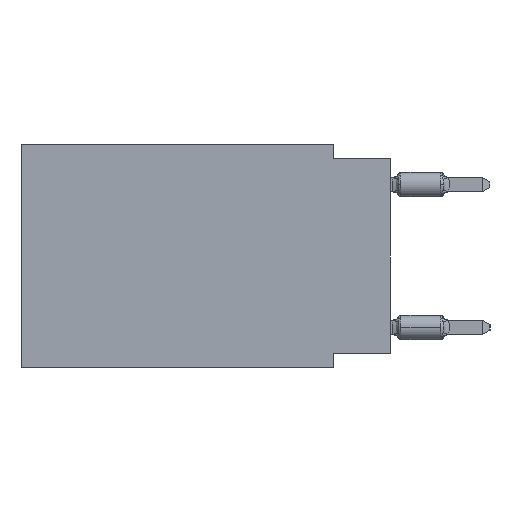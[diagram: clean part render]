
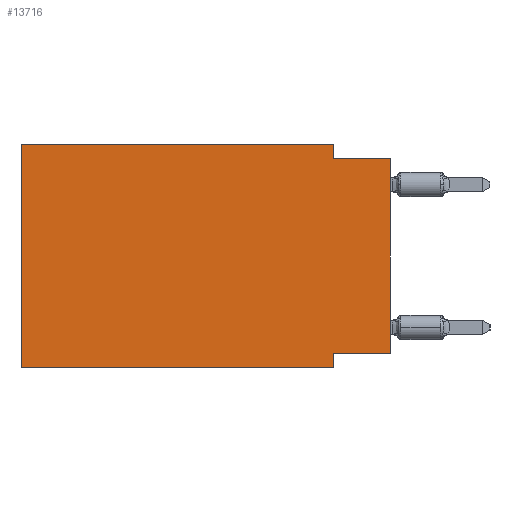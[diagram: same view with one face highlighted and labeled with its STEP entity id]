
A CAD part, left-side view. The second image highlights one B-rep face of the part: STEP entity #13716.
In plain terms, the highlighted planar face has unit normal (-1, 0, 0).
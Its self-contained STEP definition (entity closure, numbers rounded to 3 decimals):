
#2653 = VECTOR ( 'NONE', #44241, 1000. ) ;
#2977 = VECTOR ( 'NONE', #38509, 1000. ) ;
#3052 = VERTEX_POINT ( 'NONE', #7721 ) ;
#3448 = LINE ( 'NONE', #23292, #17995 ) ;
#3545 = ORIENTED_EDGE ( 'NONE', *, *, #43827, .F. ) ;
#4111 = AXIS2_PLACEMENT_3D ( 'NONE', #21947, #48461, #5827 ) ;
#4269 = VERTEX_POINT ( 'NONE', #36253 ) ;
#5827 = DIRECTION ( 'NONE',  ( 0., 0., -1. ) ) ;
#6139 = LINE ( 'NONE', #10091, #47481 ) ;
#7126 = DIRECTION ( 'NONE',  ( 0., -1., 0. ) ) ;
#7233 = VERTEX_POINT ( 'NONE', #31662 ) ;
#7721 = CARTESIAN_POINT ( 'NONE',  ( 0., 0., -9.271 ) ) ;
#7916 = CARTESIAN_POINT ( 'NONE',  ( 0., 0., 0. ) ) ;
#8437 = LINE ( 'NONE', #7916, #37009 ) ;
#9662 = DIRECTION ( 'NONE',  ( 0., -1., 0. ) ) ;
#9807 = FACE_OUTER_BOUND ( 'NONE', #15018, .T. ) ;
#10091 = CARTESIAN_POINT ( 'NONE',  ( 0., 0., -0.635 ) ) ;
#10101 = ORIENTED_EDGE ( 'NONE', *, *, #42262, .T. ) ;
#10187 = VECTOR ( 'NONE', #20282, 1000. ) ;
#10326 = CARTESIAN_POINT ( 'NONE',  ( 0., 16.383, -9.906 ) ) ;
#10565 = VERTEX_POINT ( 'NONE', #40290 ) ;
#13209 = ORIENTED_EDGE ( 'NONE', *, *, #31185, .F. ) ;
#13498 = EDGE_CURVE ( 'NONE', #15154, #10565, #43044, .T. ) ;
#13716 = ADVANCED_FACE ( 'NONE', ( #9807 ), #42030, .F. ) ;
#13750 = ORIENTED_EDGE ( 'NONE', *, *, #44589, .T. ) ;
#13898 = ORIENTED_EDGE ( 'NONE', *, *, #13498, .F. ) ;
#15018 = EDGE_LOOP ( 'NONE', ( #13750, #30929, #37680, #13898, #39206, #10101, #13209, #3545 ) ) ;
#15154 = VERTEX_POINT ( 'NONE', #19608 ) ;
#17995 = VECTOR ( 'NONE', #43879, 1000. ) ;
#18078 = VECTOR ( 'NONE', #9662, 1000. ) ;
#19608 = CARTESIAN_POINT ( 'NONE',  ( 0., 16.383, 0. ) ) ;
#20282 = DIRECTION ( 'NONE',  ( 0., 0., -1. ) ) ;
#21947 = CARTESIAN_POINT ( 'NONE',  ( 0., 16.383, 0. ) ) ;
#23292 = CARTESIAN_POINT ( 'NONE',  ( 0., 16.383, 0. ) ) ;
#26357 = CARTESIAN_POINT ( 'NONE',  ( 0., 2.54, -9.906 ) ) ;
#26955 = VERTEX_POINT ( 'NONE', #51546 ) ;
#28131 = CARTESIAN_POINT ( 'NONE',  ( 0., 0., -9.271 ) ) ;
#30258 = LINE ( 'NONE', #34238, #18078 ) ;
#30929 = ORIENTED_EDGE ( 'NONE', *, *, #50249, .F. ) ;
#31185 = EDGE_CURVE ( 'NONE', #52083, #4269, #46162, .T. ) ;
#31662 = CARTESIAN_POINT ( 'NONE',  ( 0., 2.54, -0.635 ) ) ;
#31961 = DIRECTION ( 'NONE',  ( 0., 0., 1. ) ) ;
#34238 = CARTESIAN_POINT ( 'NONE',  ( 0., 16.383, -9.906 ) ) ;
#36253 = CARTESIAN_POINT ( 'NONE',  ( 0., 2.54, -9.906 ) ) ;
#36309 = LINE ( 'NONE', #28131, #2653 ) ;
#36670 = LINE ( 'NONE', #45364, #10187 ) ;
#37009 = VECTOR ( 'NONE', #31961, 1000. ) ;
#37680 = ORIENTED_EDGE ( 'NONE', *, *, #47345, .F. ) ;
#38509 = DIRECTION ( 'NONE',  ( 0., 0., -1. ) ) ;
#39206 = ORIENTED_EDGE ( 'NONE', *, *, #41150, .F. ) ;
#39877 = CARTESIAN_POINT ( 'NONE',  ( 0., 2.54, -9.271 ) ) ;
#40290 = CARTESIAN_POINT ( 'NONE',  ( 0., 2.54, 0. ) ) ;
#41150 = EDGE_CURVE ( 'NONE', #46700, #15154, #3448, .T. ) ;
#41235 = VECTOR ( 'NONE', #7126, 1000. ) ;
#42030 = PLANE ( 'NONE',  #4111 ) ;
#42262 = EDGE_CURVE ( 'NONE', #46700, #4269, #30258, .T. ) ;
#43044 = LINE ( 'NONE', #43322, #41235 ) ;
#43322 = CARTESIAN_POINT ( 'NONE',  ( 0., 16.383, 0. ) ) ;
#43827 = EDGE_CURVE ( 'NONE', #3052, #52083, #36309, .T. ) ;
#43879 = DIRECTION ( 'NONE',  ( 0., 0., 1. ) ) ;
#44241 = DIRECTION ( 'NONE',  ( 0., 1., 0. ) ) ;
#44589 = EDGE_CURVE ( 'NONE', #3052, #26955, #8437, .T. ) ;
#45364 = CARTESIAN_POINT ( 'NONE',  ( 0., 2.54, 0. ) ) ;
#46162 = LINE ( 'NONE', #26357, #2977 ) ;
#46700 = VERTEX_POINT ( 'NONE', #10326 ) ;
#47345 = EDGE_CURVE ( 'NONE', #10565, #7233, #36670, .T. ) ;
#47481 = VECTOR ( 'NONE', #50757, 1000. ) ;
#48461 = DIRECTION ( 'NONE',  ( 1., 0., 0. ) ) ;
#50249 = EDGE_CURVE ( 'NONE', #7233, #26955, #6139, .T. ) ;
#50757 = DIRECTION ( 'NONE',  ( 0., -1., 0. ) ) ;
#51546 = CARTESIAN_POINT ( 'NONE',  ( 0., 0., -0.635 ) ) ;
#52083 = VERTEX_POINT ( 'NONE', #39877 ) ;
